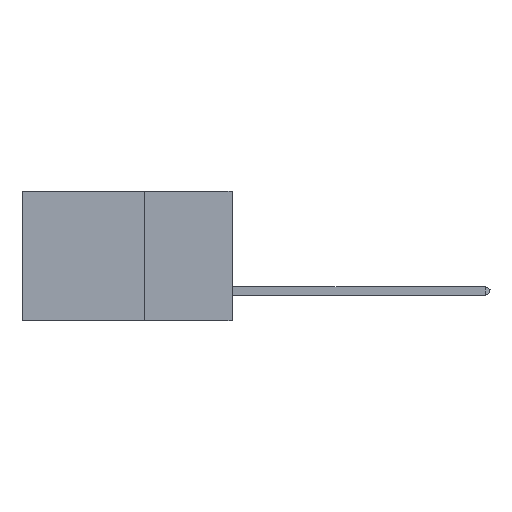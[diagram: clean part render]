
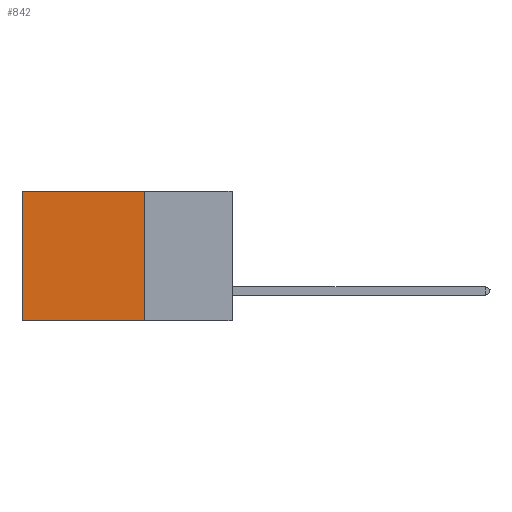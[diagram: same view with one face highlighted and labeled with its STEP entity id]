
A CAD part, left-side view. The second image highlights one B-rep face of the part: STEP entity #842.
In plain terms, the highlighted planar face has unit normal (-1, 0, 0).
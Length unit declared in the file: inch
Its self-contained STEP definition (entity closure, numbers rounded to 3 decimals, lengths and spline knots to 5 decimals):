
#763 = CARTESIAN_POINT ( 'NONE',  ( 0.2875, 0.6, -0.37 ) ) ;
#842 = ADVANCED_FACE ( 'NONE', ( #9663 ), #8773, .F. ) ;
#1636 = VECTOR ( 'NONE', #17358, 39.37008 ) ;
#1685 = CARTESIAN_POINT ( 'NONE',  ( 0.2875, 0.25, 0. ) ) ;
#2000 = AXIS2_PLACEMENT_3D ( 'NONE', #13041, #17399, #8895 ) ;
#2025 = VERTEX_POINT ( 'NONE', #763 ) ;
#2819 = VECTOR ( 'NONE', #10081, 39.37008 ) ;
#3436 = EDGE_CURVE ( 'NONE', #11782, #2025, #14336, .T. ) ;
#4342 = LINE ( 'NONE', #1685, #1636 ) ;
#4889 = DIRECTION ( 'NONE',  ( 0., 1., 0. ) ) ;
#5791 = VECTOR ( 'NONE', #4889, 39.37008 ) ;
#6137 = EDGE_CURVE ( 'NONE', #9612, #2025, #14887, .T. ) ;
#7072 = ORIENTED_EDGE ( 'NONE', *, *, #3436, .T. ) ;
#8773 = PLANE ( 'NONE',  #2000 ) ;
#8895 = DIRECTION ( 'NONE',  ( 0., 0., -1. ) ) ;
#9612 = VERTEX_POINT ( 'NONE', #13828 ) ;
#9663 = FACE_OUTER_BOUND ( 'NONE', #15091, .T. ) ;
#10081 = DIRECTION ( 'NONE',  ( 0., 1., 0. ) ) ;
#11030 = LINE ( 'NONE', #16062, #2819 ) ;
#11073 = DIRECTION ( 'NONE',  ( 0., 0., -1. ) ) ;
#11782 = VERTEX_POINT ( 'NONE', #13555 ) ;
#13041 = CARTESIAN_POINT ( 'NONE',  ( 0.2875, 0.25, 0. ) ) ;
#13555 = CARTESIAN_POINT ( 'NONE',  ( 0.2875, 0.6, 0. ) ) ;
#13828 = CARTESIAN_POINT ( 'NONE',  ( 0.2875, 0.25, -0.37 ) ) ;
#14336 = LINE ( 'NONE', #16736, #17647 ) ;
#14415 = ORIENTED_EDGE ( 'NONE', *, *, #15559, .T. ) ;
#14649 = VERTEX_POINT ( 'NONE', #14883 ) ;
#14883 = CARTESIAN_POINT ( 'NONE',  ( 0.2875, 0.25, 0. ) ) ;
#14887 = LINE ( 'NONE', #17609, #5791 ) ;
#15091 = EDGE_LOOP ( 'NONE', ( #7072, #16081, #18171, #14415 ) ) ;
#15559 = EDGE_CURVE ( 'NONE', #14649, #11782, #11030, .T. ) ;
#16062 = CARTESIAN_POINT ( 'NONE',  ( 0.2875, 0.25, 0. ) ) ;
#16081 = ORIENTED_EDGE ( 'NONE', *, *, #6137, .F. ) ;
#16736 = CARTESIAN_POINT ( 'NONE',  ( 0.2875, 0.6, 0. ) ) ;
#17337 = EDGE_CURVE ( 'NONE', #14649, #9612, #4342, .T. ) ;
#17358 = DIRECTION ( 'NONE',  ( 0., 0., -1. ) ) ;
#17399 = DIRECTION ( 'NONE',  ( 1., 0., 0. ) ) ;
#17609 = CARTESIAN_POINT ( 'NONE',  ( 0.2875, 0.25, -0.37 ) ) ;
#17647 = VECTOR ( 'NONE', #11073, 39.37008 ) ;
#18171 = ORIENTED_EDGE ( 'NONE', *, *, #17337, .F. ) ;
